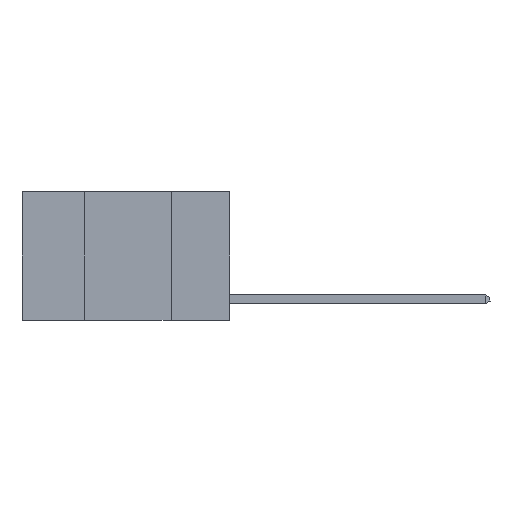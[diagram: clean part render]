
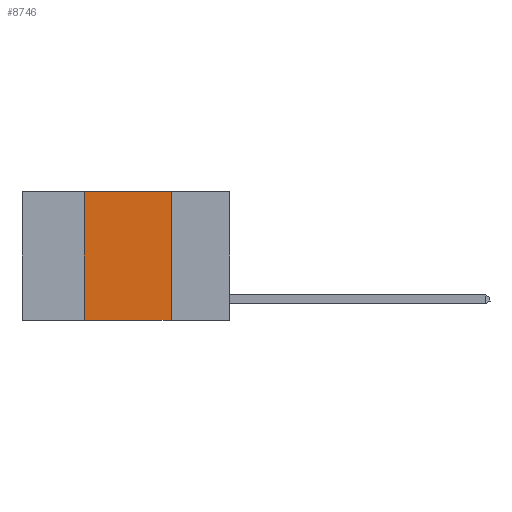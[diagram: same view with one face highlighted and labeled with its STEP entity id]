
A CAD part, left-side view. The second image highlights one B-rep face of the part: STEP entity #8746.
In plain terms, the highlighted planar face has unit normal (-1, 0, 0).
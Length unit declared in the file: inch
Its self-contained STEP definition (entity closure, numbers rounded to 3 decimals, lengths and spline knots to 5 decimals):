
#284 = VECTOR ( 'NONE', #2667, 39.37008 ) ;
#986 = CARTESIAN_POINT ( 'NONE',  ( 0., 0.6, -0.37 ) ) ;
#1726 = AXIS2_PLACEMENT_3D ( 'NONE', #13934, #20680, #7341 ) ;
#1884 = ORIENTED_EDGE ( 'NONE', *, *, #8694, .F. ) ;
#2667 = DIRECTION ( 'NONE',  ( 0., -1., 0. ) ) ;
#2859 = EDGE_CURVE ( 'NONE', #14260, #7099, #16089, .T. ) ;
#2867 = PLANE ( 'NONE',  #1726 ) ;
#2926 = DIRECTION ( 'NONE',  ( 0., 0., -1. ) ) ;
#3436 = CARTESIAN_POINT ( 'NONE',  ( 0., 0.17, -0.37 ) ) ;
#3971 = EDGE_CURVE ( 'NONE', #21279, #7099, #15336, .T. ) ;
#5480 = DIRECTION ( 'NONE',  ( 0., -1., 0. ) ) ;
#5534 = CARTESIAN_POINT ( 'NONE',  ( 0., 0.42, -0.37 ) ) ;
#6219 = LINE ( 'NONE', #22652, #284 ) ;
#6416 = ORIENTED_EDGE ( 'NONE', *, *, #2859, .F. ) ;
#7099 = VERTEX_POINT ( 'NONE', #3436 ) ;
#7341 = DIRECTION ( 'NONE',  ( 0., 0., -1. ) ) ;
#7393 = CARTESIAN_POINT ( 'NONE',  ( 0., 0.17, 0. ) ) ;
#8694 = EDGE_CURVE ( 'NONE', #27822, #14260, #6219, .T. ) ;
#8746 = ADVANCED_FACE ( 'NONE', ( #27824 ), #2867, .F. ) ;
#9482 = VECTOR ( 'NONE', #2926, 39.37008 ) ;
#9586 = VECTOR ( 'NONE', #22332, 39.37008 ) ;
#12384 = EDGE_LOOP ( 'NONE', ( #6416, #1884, #14406, #15806 ) ) ;
#13934 = CARTESIAN_POINT ( 'NONE',  ( 0., 0.6, 0. ) ) ;
#14260 = VERTEX_POINT ( 'NONE', #28426 ) ;
#14406 = ORIENTED_EDGE ( 'NONE', *, *, #27675, .F. ) ;
#15336 = LINE ( 'NONE', #986, #26530 ) ;
#15806 = ORIENTED_EDGE ( 'NONE', *, *, #3971, .T. ) ;
#16089 = LINE ( 'NONE', #7393, #9482 ) ;
#20680 = DIRECTION ( 'NONE',  ( 1., 0., 0. ) ) ;
#21279 = VERTEX_POINT ( 'NONE', #5534 ) ;
#22332 = DIRECTION ( 'NONE',  ( 0., 0., 1. ) ) ;
#22652 = CARTESIAN_POINT ( 'NONE',  ( 0., 0.6, 0. ) ) ;
#24457 = CARTESIAN_POINT ( 'NONE',  ( 0., 0.42, 0. ) ) ;
#25040 = CARTESIAN_POINT ( 'NONE',  ( 0., 0.42, 0. ) ) ;
#26530 = VECTOR ( 'NONE', #5480, 39.37008 ) ;
#27675 = EDGE_CURVE ( 'NONE', #21279, #27822, #28738, .T. ) ;
#27822 = VERTEX_POINT ( 'NONE', #25040 ) ;
#27824 = FACE_OUTER_BOUND ( 'NONE', #12384, .T. ) ;
#28426 = CARTESIAN_POINT ( 'NONE',  ( 0., 0.17, 0. ) ) ;
#28738 = LINE ( 'NONE', #24457, #9586 ) ;
